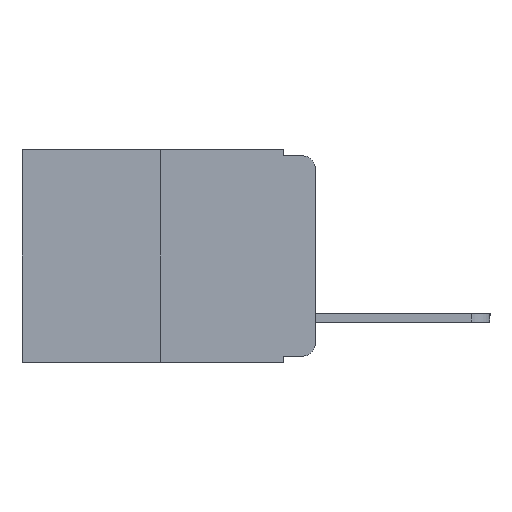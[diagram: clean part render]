
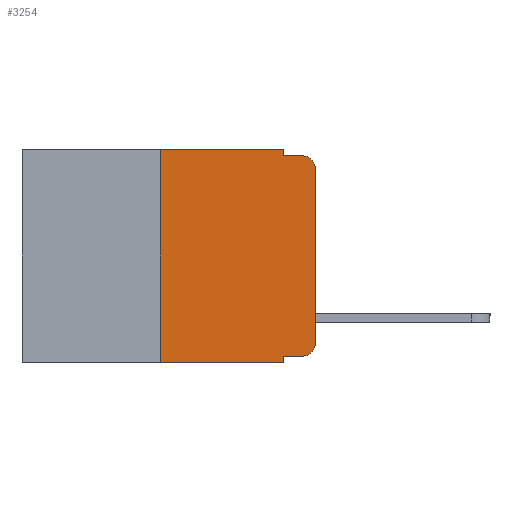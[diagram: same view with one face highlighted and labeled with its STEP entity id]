
A CAD part, left-side view. The second image highlights one B-rep face of the part: STEP entity #3254.
In plain terms, the highlighted planar face has unit normal (-1, 0, 0).
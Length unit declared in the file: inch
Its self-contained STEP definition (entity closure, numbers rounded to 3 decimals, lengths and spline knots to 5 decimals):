
#260 = CARTESIAN_POINT ( 'NONE',  ( 0., 0.473, -0.343 ) ) ;
#534 = DIRECTION ( 'NONE',  ( 0., -1., 0. ) ) ;
#1067 = DIRECTION ( 'NONE',  ( 0., 0., -1. ) ) ;
#1173 = LINE ( 'NONE', #6139, #4517 ) ;
#1425 = CARTESIAN_POINT ( 'NONE',  ( 0., 0.051, -0.333 ) ) ;
#1574 = EDGE_CURVE ( 'NONE', #9598, #3687, #14254, .T. ) ;
#1596 = EDGE_CURVE ( 'NONE', #4265, #14721, #1173, .T. ) ;
#1645 = ORIENTED_EDGE ( 'NONE', *, *, #1574, .F. ) ;
#1893 = DIRECTION ( 'NONE',  ( 0., 0., -1. ) ) ;
#2165 = EDGE_CURVE ( 'NONE', #13627, #9204, #10715, .T. ) ;
#2330 = ORIENTED_EDGE ( 'NONE', *, *, #2165, .T. ) ;
#3064 = ORIENTED_EDGE ( 'NONE', *, *, #5202, .T. ) ;
#3254 = ADVANCED_FACE ( 'NONE', ( #6700 ), #15126, .F. ) ;
#3278 = CARTESIAN_POINT ( 'NONE',  ( 0., 0.25, 0. ) ) ;
#3283 = ORIENTED_EDGE ( 'NONE', *, *, #6102, .T. ) ;
#3687 = VERTEX_POINT ( 'NONE', #10960 ) ;
#3725 = CARTESIAN_POINT ( 'NONE',  ( 0., 0.02, -0.03 ) ) ;
#4039 = ORIENTED_EDGE ( 'NONE', *, *, #13197, .F. ) ;
#4265 = VERTEX_POINT ( 'NONE', #5023 ) ;
#4451 = DIRECTION ( 'NONE',  ( 0., 0., -1. ) ) ;
#4517 = VECTOR ( 'NONE', #534, 39.37008 ) ;
#4560 = VERTEX_POINT ( 'NONE', #12692 ) ;
#4772 = CARTESIAN_POINT ( 'NONE',  ( 0., 0., -0.03 ) ) ;
#5023 = CARTESIAN_POINT ( 'NONE',  ( 0., 0.051, -0.01 ) ) ;
#5103 = DIRECTION ( 'NONE',  ( 0., 0., -1. ) ) ;
#5183 = DIRECTION ( 'NONE',  ( 0., 0., 1. ) ) ;
#5202 = EDGE_CURVE ( 'NONE', #7928, #4560, #14435, .T. ) ;
#5333 = AXIS2_PLACEMENT_3D ( 'NONE', #15628, #8889, #1067 ) ;
#5396 = CARTESIAN_POINT ( 'NONE',  ( 0., 0.02, -0.333 ) ) ;
#5652 = AXIS2_PLACEMENT_3D ( 'NONE', #8385, #9513, #1893 ) ;
#6102 = EDGE_CURVE ( 'NONE', #13213, #7928, #8572, .T. ) ;
#6139 = CARTESIAN_POINT ( 'NONE',  ( 0., 0.051, -0.01 ) ) ;
#6358 = VECTOR ( 'NONE', #4451, 39.37008 ) ;
#6700 = FACE_OUTER_BOUND ( 'NONE', #8175, .T. ) ;
#6843 = CARTESIAN_POINT ( 'NONE',  ( 0., 0.051, 0. ) ) ;
#6892 = EDGE_CURVE ( 'NONE', #13213, #9204, #7107, .T. ) ;
#7057 = CARTESIAN_POINT ( 'NONE',  ( 0., 0.051, 0. ) ) ;
#7107 = LINE ( 'NONE', #7057, #6358 ) ;
#7228 = EDGE_CURVE ( 'NONE', #12783, #14721, #14542, .T. ) ;
#7695 = CARTESIAN_POINT ( 'NONE',  ( 0., 0.02, -0.01 ) ) ;
#7928 = VERTEX_POINT ( 'NONE', #5396 ) ;
#7936 = CARTESIAN_POINT ( 'NONE',  ( 0., 0., 0. ) ) ;
#8040 = DIRECTION ( 'NONE',  ( 0., 0., -1. ) ) ;
#8163 = DIRECTION ( 'NONE',  ( 0., -1., 0. ) ) ;
#8175 = EDGE_LOOP ( 'NONE', ( #9242, #12092, #12178, #4039, #1645, #12512, #2330, #8581, #3283, #3064 ) ) ;
#8385 = CARTESIAN_POINT ( 'NONE',  ( 0., 0.473, 0. ) ) ;
#8572 = LINE ( 'NONE', #11614, #11255 ) ;
#8581 = ORIENTED_EDGE ( 'NONE', *, *, #6892, .F. ) ;
#8749 = CARTESIAN_POINT ( 'NONE',  ( 0., 0.473, 0. ) ) ;
#8761 = CARTESIAN_POINT ( 'NONE',  ( 0., 0.25, 0. ) ) ;
#8803 = CARTESIAN_POINT ( 'NONE',  ( 0., 0.051, -0.343 ) ) ;
#8889 = DIRECTION ( 'NONE',  ( -1., 0., 0. ) ) ;
#9176 = DIRECTION ( 'NONE',  ( 0., -1., 0. ) ) ;
#9204 = VERTEX_POINT ( 'NONE', #8803 ) ;
#9242 = ORIENTED_EDGE ( 'NONE', *, *, #15596, .T. ) ;
#9347 = AXIS2_PLACEMENT_3D ( 'NONE', #3725, #12190, #5103 ) ;
#9513 = DIRECTION ( 'NONE',  ( 1., 0., 0. ) ) ;
#9598 = VERTEX_POINT ( 'NONE', #3278 ) ;
#10341 = VECTOR ( 'NONE', #12552, 39.37008 ) ;
#10715 = LINE ( 'NONE', #260, #10341 ) ;
#10764 = VECTOR ( 'NONE', #15726, 39.37008 ) ;
#10960 = CARTESIAN_POINT ( 'NONE',  ( 0., 0.051, 0. ) ) ;
#11122 = LINE ( 'NONE', #7936, #10764 ) ;
#11255 = VECTOR ( 'NONE', #8163, 39.37008 ) ;
#11614 = CARTESIAN_POINT ( 'NONE',  ( 0., 0.051, -0.333 ) ) ;
#12092 = ORIENTED_EDGE ( 'NONE', *, *, #7228, .T. ) ;
#12178 = ORIENTED_EDGE ( 'NONE', *, *, #1596, .F. ) ;
#12189 = CARTESIAN_POINT ( 'NONE',  ( 0., 0.25, -0.343 ) ) ;
#12190 = DIRECTION ( 'NONE',  ( -1., 0., 0. ) ) ;
#12512 = ORIENTED_EDGE ( 'NONE', *, *, #12978, .F. ) ;
#12552 = DIRECTION ( 'NONE',  ( 0., -1., 0. ) ) ;
#12692 = CARTESIAN_POINT ( 'NONE',  ( 0., 0., -0.313 ) ) ;
#12783 = VERTEX_POINT ( 'NONE', #4772 ) ;
#12978 = EDGE_CURVE ( 'NONE', #13627, #9598, #15865, .T. ) ;
#13161 = LINE ( 'NONE', #6843, #15691 ) ;
#13197 = EDGE_CURVE ( 'NONE', #3687, #4265, #13161, .T. ) ;
#13213 = VERTEX_POINT ( 'NONE', #1425 ) ;
#13627 = VERTEX_POINT ( 'NONE', #12189 ) ;
#13905 = VECTOR ( 'NONE', #9176, 39.37008 ) ;
#14254 = LINE ( 'NONE', #8749, #13905 ) ;
#14435 = CIRCLE ( 'NONE', #5333, 0.02 ) ;
#14542 = CIRCLE ( 'NONE', #9347, 0.02 ) ;
#14721 = VERTEX_POINT ( 'NONE', #7695 ) ;
#15126 = PLANE ( 'NONE',  #5652 ) ;
#15197 = VECTOR ( 'NONE', #5183, 39.37008 ) ;
#15596 = EDGE_CURVE ( 'NONE', #4560, #12783, #11122, .T. ) ;
#15628 = CARTESIAN_POINT ( 'NONE',  ( 0., 0.02, -0.313 ) ) ;
#15691 = VECTOR ( 'NONE', #8040, 39.37008 ) ;
#15726 = DIRECTION ( 'NONE',  ( 0., 0., 1. ) ) ;
#15865 = LINE ( 'NONE', #8761, #15197 ) ;
